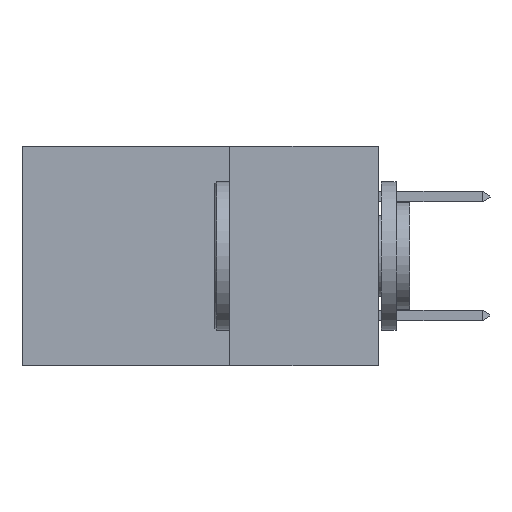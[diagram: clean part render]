
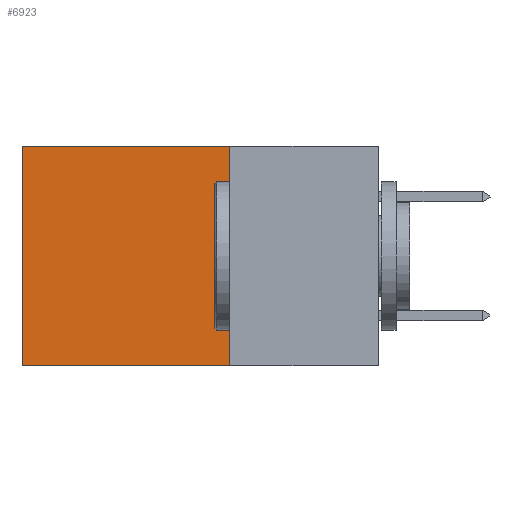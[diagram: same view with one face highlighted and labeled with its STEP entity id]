
A CAD part, left-side view. The second image highlights one B-rep face of the part: STEP entity #6923.
In plain terms, the highlighted planar face has unit normal (-1, 0, 0).
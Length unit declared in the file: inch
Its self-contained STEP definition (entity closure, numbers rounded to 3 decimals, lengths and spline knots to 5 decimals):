
#208 = CARTESIAN_POINT ( 'NONE',  ( 0.298, 0.6, 0. ) ) ;
#299 = CARTESIAN_POINT ( 'NONE',  ( 0.298, 0.25, 0. ) ) ;
#1017 = VERTEX_POINT ( 'NONE', #299 ) ;
#1034 = VECTOR ( 'NONE', #4805, 39.37008 ) ;
#1174 = LINE ( 'NONE', #11384, #1034 ) ;
#1313 = DIRECTION ( 'NONE',  ( 1., 0., 0. ) ) ;
#1785 = VERTEX_POINT ( 'NONE', #208 ) ;
#2350 = DIRECTION ( 'NONE',  ( 0., 0., -1. ) ) ;
#2461 = LINE ( 'NONE', #4877, #4421 ) ;
#2491 = VERTEX_POINT ( 'NONE', #10017 ) ;
#2530 = VERTEX_POINT ( 'NONE', #3490 ) ;
#2654 = EDGE_LOOP ( 'NONE', ( #11031, #6106, #4976, #7235 ) ) ;
#2778 = EDGE_CURVE ( 'NONE', #1785, #2491, #1174, .T. ) ;
#3131 = LINE ( 'NONE', #5399, #10425 ) ;
#3490 = CARTESIAN_POINT ( 'NONE',  ( 0.298, 0.25, -0.37 ) ) ;
#4035 = FACE_OUTER_BOUND ( 'NONE', #2654, .T. ) ;
#4421 = VECTOR ( 'NONE', #11947, 39.37008 ) ;
#4805 = DIRECTION ( 'NONE',  ( 0., 0., -1. ) ) ;
#4877 = CARTESIAN_POINT ( 'NONE',  ( 0.298, 0.25, 0. ) ) ;
#4916 = DIRECTION ( 'NONE',  ( 0., 1., 0. ) ) ;
#4976 = ORIENTED_EDGE ( 'NONE', *, *, #6632, .F. ) ;
#5399 = CARTESIAN_POINT ( 'NONE',  ( 0.298, 0.25, 0. ) ) ;
#5589 = LINE ( 'NONE', #11846, #10430 ) ;
#6106 = ORIENTED_EDGE ( 'NONE', *, *, #12172, .F. ) ;
#6632 = EDGE_CURVE ( 'NONE', #1017, #2530, #3131, .T. ) ;
#6923 = ADVANCED_FACE ( 'NONE', ( #4035 ), #8359, .F. ) ;
#7235 = ORIENTED_EDGE ( 'NONE', *, *, #9087, .T. ) ;
#8359 = PLANE ( 'NONE',  #8835 ) ;
#8835 = AXIS2_PLACEMENT_3D ( 'NONE', #12048, #1313, #2350 ) ;
#9087 = EDGE_CURVE ( 'NONE', #1017, #1785, #2461, .T. ) ;
#10017 = CARTESIAN_POINT ( 'NONE',  ( 0.298, 0.6, -0.37 ) ) ;
#10425 = VECTOR ( 'NONE', #11111, 39.37008 ) ;
#10430 = VECTOR ( 'NONE', #4916, 39.37008 ) ;
#11031 = ORIENTED_EDGE ( 'NONE', *, *, #2778, .T. ) ;
#11111 = DIRECTION ( 'NONE',  ( 0., 0., -1. ) ) ;
#11384 = CARTESIAN_POINT ( 'NONE',  ( 0.298, 0.6, 0. ) ) ;
#11846 = CARTESIAN_POINT ( 'NONE',  ( 0.298, 0.25, -0.37 ) ) ;
#11947 = DIRECTION ( 'NONE',  ( 0., 1., 0. ) ) ;
#12048 = CARTESIAN_POINT ( 'NONE',  ( 0.298, 0.25, 0. ) ) ;
#12172 = EDGE_CURVE ( 'NONE', #2530, #2491, #5589, .T. ) ;
